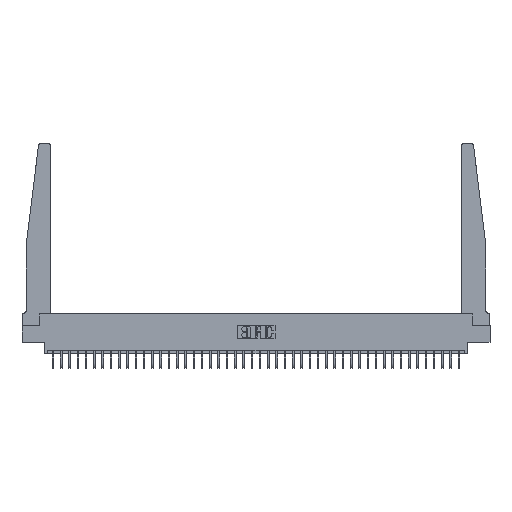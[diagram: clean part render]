
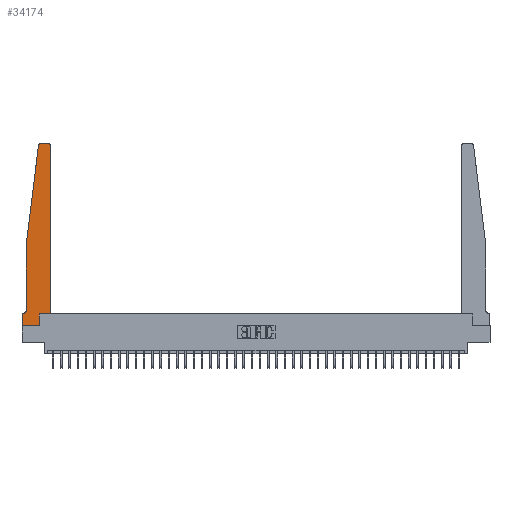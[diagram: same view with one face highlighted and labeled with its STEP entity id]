
A CAD part, top view. The second image highlights one B-rep face of the part: STEP entity #34174.
In plain terms, the highlighted planar face has unit normal (0, 0, 1).
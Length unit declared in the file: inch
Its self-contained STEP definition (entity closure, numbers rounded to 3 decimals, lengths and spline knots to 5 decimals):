
#120 = ORIENTED_EDGE ( 'NONE', *, *, #14108, .T. ) ;
#283 = CARTESIAN_POINT ( 'NONE',  ( 0.015, 0.2375, 0.37 ) ) ;
#317 = VECTOR ( 'NONE', #29202, 39.37008 ) ;
#669 = VERTEX_POINT ( 'NONE', #11240 ) ;
#695 = CARTESIAN_POINT ( 'NONE',  ( 0.395, 2.75, 0.37 ) ) ;
#767 = CIRCLE ( 'NONE', #28293, 0.05 ) ;
#1143 = DIRECTION ( 'NONE',  ( 1., 0., 0. ) ) ;
#1207 = CARTESIAN_POINT ( 'NONE',  ( 0.425, 0.18, 0.37 ) ) ;
#1227 = DIRECTION ( 'NONE',  ( 0., 0., 1. ) ) ;
#1657 = EDGE_CURVE ( 'NONE', #5508, #31542, #767, .T. ) ;
#1803 = ORIENTED_EDGE ( 'NONE', *, *, #23543, .T. ) ;
#2320 = ORIENTED_EDGE ( 'NONE', *, *, #29881, .T. ) ;
#3660 = CARTESIAN_POINT ( 'NONE',  ( 0., 0., 0.37 ) ) ;
#4134 = LINE ( 'NONE', #16100, #5307 ) ;
#4672 = DIRECTION ( 'NONE',  ( 0., 1., 0. ) ) ;
#5207 = ORIENTED_EDGE ( 'NONE', *, *, #22971, .T. ) ;
#5268 = DIRECTION ( 'NONE',  ( 0., -1., 0. ) ) ;
#5307 = VECTOR ( 'NONE', #16494, 39.37008 ) ;
#5392 = CARTESIAN_POINT ( 'NONE',  ( 0.27653, 2.72, 0.37 ) ) ;
#5508 = VERTEX_POINT ( 'NONE', #11072 ) ;
#5589 = LINE ( 'NONE', #29494, #31500 ) ;
#6087 = AXIS2_PLACEMENT_3D ( 'NONE', #5392, #25971, #7925 ) ;
#6088 = ORIENTED_EDGE ( 'NONE', *, *, #17834, .T. ) ;
#6192 = EDGE_CURVE ( 'NONE', #21016, #669, #21170, .T. ) ;
#6739 = VERTEX_POINT ( 'NONE', #36760 ) ;
#6789 = EDGE_CURVE ( 'NONE', #9606, #35244, #7721, .T. ) ;
#7329 = VECTOR ( 'NONE', #5268, 39.37008 ) ;
#7721 = LINE ( 'NONE', #3660, #21433 ) ;
#7925 = DIRECTION ( 'NONE',  ( 1., 0., 0. ) ) ;
#9541 = DIRECTION ( 'NONE',  ( 0., -1., 0. ) ) ;
#9606 = VERTEX_POINT ( 'NONE', #28572 ) ;
#9940 = CARTESIAN_POINT ( 'NONE',  ( 0., 0., 0.37 ) ) ;
#9953 = VERTEX_POINT ( 'NONE', #695 ) ;
#10456 = EDGE_CURVE ( 'NONE', #37772, #11905, #12966, .T. ) ;
#10536 = CARTESIAN_POINT ( 'NONE',  ( 0.425, 0.18, 0.37 ) ) ;
#11072 = CARTESIAN_POINT ( 'NONE',  ( 0.065, 0.2375, 0.37 ) ) ;
#11240 = CARTESIAN_POINT ( 'NONE',  ( 0.425, 2.72, 0.37 ) ) ;
#11350 = CARTESIAN_POINT ( 'NONE',  ( 0., 0., 0.37 ) ) ;
#11546 = CARTESIAN_POINT ( 'NONE',  ( 0.065, 1.25, 0.37 ) ) ;
#11905 = VERTEX_POINT ( 'NONE', #25976 ) ;
#12242 = DIRECTION ( 'NONE',  ( 0., 0., -1. ) ) ;
#12966 = CIRCLE ( 'NONE', #6087, 0.03 ) ;
#13048 = ORIENTED_EDGE ( 'NONE', *, *, #1657, .T. ) ;
#14108 = EDGE_CURVE ( 'NONE', #669, #9953, #23200, .T. ) ;
#14718 = DIRECTION ( 'NONE',  ( 0., 1., 0. ) ) ;
#15283 = CARTESIAN_POINT ( 'NONE',  ( 0.425, 0.18, 0.37 ) ) ;
#15557 = DIRECTION ( 'NONE',  ( -1., 0., 0. ) ) ;
#16100 = CARTESIAN_POINT ( 'NONE',  ( 0.065, 1.25, 0.37 ) ) ;
#16117 = DIRECTION ( 'NONE',  ( 1., 0., 0. ) ) ;
#16494 = DIRECTION ( 'NONE',  ( -0.122, -0.992, 0. ) ) ;
#16608 = VECTOR ( 'NONE', #4672, 39.37008 ) ;
#17659 = CARTESIAN_POINT ( 'NONE',  ( 0.395, 2.72, 0.37 ) ) ;
#17834 = EDGE_CURVE ( 'NONE', #29906, #21016, #37267, .T. ) ;
#18302 = ORIENTED_EDGE ( 'NONE', *, *, #6789, .T. ) ;
#18670 = ORIENTED_EDGE ( 'NONE', *, *, #30419, .T. ) ;
#18866 = CARTESIAN_POINT ( 'NONE',  ( 0.27653, 2.75, 0.37 ) ) ;
#18886 = PLANE ( 'NONE',  #21059 ) ;
#19089 = FACE_OUTER_BOUND ( 'NONE', #25918, .T. ) ;
#19993 = CARTESIAN_POINT ( 'NONE',  ( 0.25, 2.75, 0.37 ) ) ;
#20505 = ORIENTED_EDGE ( 'NONE', *, *, #32960, .T. ) ;
#20677 = DIRECTION ( 'NONE',  ( -1., 0., 0. ) ) ;
#20969 = DIRECTION ( 'NONE',  ( 0., 0., 1. ) ) ;
#21016 = VERTEX_POINT ( 'NONE', #10536 ) ;
#21059 = AXIS2_PLACEMENT_3D ( 'NONE', #28079, #1227, #29013 ) ;
#21170 = LINE ( 'NONE', #15283, #26541 ) ;
#21433 = VECTOR ( 'NONE', #9541, 39.37008 ) ;
#22529 = CARTESIAN_POINT ( 'NONE',  ( 0.015, 0.1875, 0.37 ) ) ;
#22971 = EDGE_CURVE ( 'NONE', #11905, #6739, #4134, .T. ) ;
#23200 = CIRCLE ( 'NONE', #32557, 0.03 ) ;
#23369 = ORIENTED_EDGE ( 'NONE', *, *, #35300, .T. ) ;
#23543 = EDGE_CURVE ( 'NONE', #28363, #29906, #31909, .T. ) ;
#25918 = EDGE_LOOP ( 'NONE', ( #20505, #34208, #5207, #23369, #13048, #2320, #18302, #18670, #1803, #6088, #33826, #120 ) ) ;
#25971 = DIRECTION ( 'NONE',  ( 0., 0., 1. ) ) ;
#25976 = CARTESIAN_POINT ( 'NONE',  ( 0.24675, 2.72367, 0.37 ) ) ;
#26541 = VECTOR ( 'NONE', #14718, 39.37008 ) ;
#28079 = CARTESIAN_POINT ( 'NONE',  ( 0., 0.1875, 0.37 ) ) ;
#28293 = AXIS2_PLACEMENT_3D ( 'NONE', #283, #12242, #15557 ) ;
#28363 = VERTEX_POINT ( 'NONE', #31619 ) ;
#28572 = CARTESIAN_POINT ( 'NONE',  ( 0., 0.1875, 0.37 ) ) ;
#29013 = DIRECTION ( 'NONE',  ( 1., 0., 0. ) ) ;
#29202 = DIRECTION ( 'NONE',  ( -1., 0., 0. ) ) ;
#29494 = CARTESIAN_POINT ( 'NONE',  ( 0.065, 0.1875, 0.37 ) ) ;
#29600 = DIRECTION ( 'NONE',  ( 1., 0., 0. ) ) ;
#29760 = LINE ( 'NONE', #11546, #7329 ) ;
#29881 = EDGE_CURVE ( 'NONE', #31542, #9606, #5589, .T. ) ;
#29906 = VERTEX_POINT ( 'NONE', #35374 ) ;
#30419 = EDGE_CURVE ( 'NONE', #35244, #28363, #36787, .T. ) ;
#31500 = VECTOR ( 'NONE', #20677, 39.37008 ) ;
#31542 = VERTEX_POINT ( 'NONE', #22529 ) ;
#31619 = CARTESIAN_POINT ( 'NONE',  ( 0.2605, 0., 0.37 ) ) ;
#31909 = LINE ( 'NONE', #34452, #16608 ) ;
#32026 = VECTOR ( 'NONE', #16117, 39.37008 ) ;
#32557 = AXIS2_PLACEMENT_3D ( 'NONE', #17659, #20969, #29600 ) ;
#32960 = EDGE_CURVE ( 'NONE', #9953, #37772, #34877, .T. ) ;
#33826 = ORIENTED_EDGE ( 'NONE', *, *, #6192, .T. ) ;
#34174 = ADVANCED_FACE ( 'NONE', ( #19089 ), #18886, .T. ) ;
#34208 = ORIENTED_EDGE ( 'NONE', *, *, #10456, .T. ) ;
#34452 = CARTESIAN_POINT ( 'NONE',  ( 0.2605, 0.18, 0.37 ) ) ;
#34877 = LINE ( 'NONE', #19993, #317 ) ;
#35244 = VERTEX_POINT ( 'NONE', #11350 ) ;
#35300 = EDGE_CURVE ( 'NONE', #6739, #5508, #29760, .T. ) ;
#35374 = CARTESIAN_POINT ( 'NONE',  ( 0.2605, 0.18, 0.37 ) ) ;
#36501 = VECTOR ( 'NONE', #1143, 39.37008 ) ;
#36760 = CARTESIAN_POINT ( 'NONE',  ( 0.065, 1.25, 0.37 ) ) ;
#36787 = LINE ( 'NONE', #9940, #36501 ) ;
#37267 = LINE ( 'NONE', #1207, #32026 ) ;
#37772 = VERTEX_POINT ( 'NONE', #18866 ) ;
